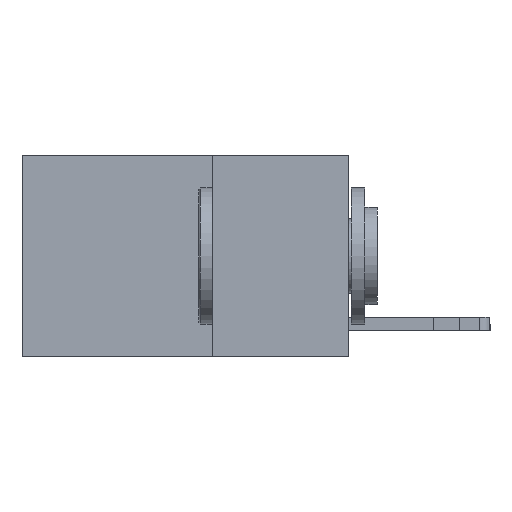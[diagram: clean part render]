
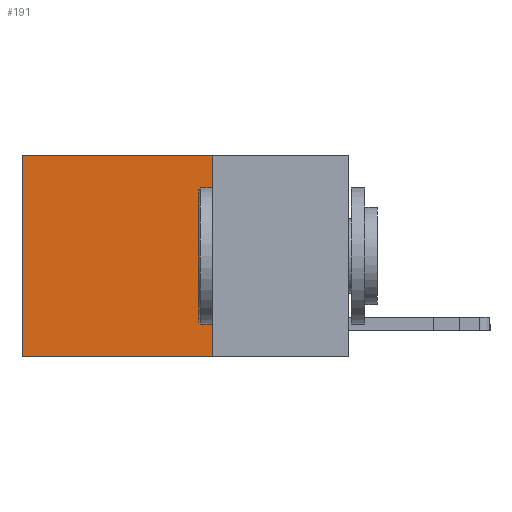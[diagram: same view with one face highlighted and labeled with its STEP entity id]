
A CAD part, left-side view. The second image highlights one B-rep face of the part: STEP entity #191.
In plain terms, the highlighted planar face has unit normal (-1, 0, 0).
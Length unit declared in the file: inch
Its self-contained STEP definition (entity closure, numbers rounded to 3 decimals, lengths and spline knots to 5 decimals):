
#33 = PLANE ( 'NONE',  #14821 ) ;
#191 = ADVANCED_FACE ( 'NONE', ( #10286 ), #33, .F. ) ;
#296 = CARTESIAN_POINT ( 'NONE',  ( 0.2625, 0.25, 0. ) ) ;
#1462 = DIRECTION ( 'NONE',  ( 0., 0., -1. ) ) ;
#2410 = CARTESIAN_POINT ( 'NONE',  ( 0.2625, 0.6, 0. ) ) ;
#2831 = DIRECTION ( 'NONE',  ( 0., 0., -1. ) ) ;
#4103 = CARTESIAN_POINT ( 'NONE',  ( 0.2625, 0.25, -0.37 ) ) ;
#4836 = ORIENTED_EDGE ( 'NONE', *, *, #6545, .F. ) ;
#4882 = DIRECTION ( 'NONE',  ( 1., 0., 0. ) ) ;
#6545 = EDGE_CURVE ( 'NONE', #16766, #10896, #7653, .T. ) ;
#7653 = LINE ( 'NONE', #4103, #22746 ) ;
#8190 = VECTOR ( 'NONE', #2831, 39.37008 ) ;
#8811 = CARTESIAN_POINT ( 'NONE',  ( 0.2625, 0.6, 0. ) ) ;
#8828 = ORIENTED_EDGE ( 'NONE', *, *, #20464, .T. ) ;
#9336 = CARTESIAN_POINT ( 'NONE',  ( 0.2625, 0.6, -0.37 ) ) ;
#9609 = CARTESIAN_POINT ( 'NONE',  ( 0.2625, 0.25, 0. ) ) ;
#9958 = LINE ( 'NONE', #9609, #13652 ) ;
#10286 = FACE_OUTER_BOUND ( 'NONE', #22119, .T. ) ;
#10896 = VERTEX_POINT ( 'NONE', #9336 ) ;
#12114 = VERTEX_POINT ( 'NONE', #296 ) ;
#12209 = LINE ( 'NONE', #8811, #22884 ) ;
#12689 = EDGE_CURVE ( 'NONE', #12114, #16766, #16728, .T. ) ;
#13377 = ORIENTED_EDGE ( 'NONE', *, *, #12689, .F. ) ;
#13652 = VECTOR ( 'NONE', #20210, 39.37008 ) ;
#14283 = CARTESIAN_POINT ( 'NONE',  ( 0.2625, 0.25, 0. ) ) ;
#14821 = AXIS2_PLACEMENT_3D ( 'NONE', #14283, #4882, #1462 ) ;
#16728 = LINE ( 'NONE', #20826, #8190 ) ;
#16766 = VERTEX_POINT ( 'NONE', #20077 ) ;
#17743 = DIRECTION ( 'NONE',  ( 0., 0., -1. ) ) ;
#19477 = ORIENTED_EDGE ( 'NONE', *, *, #21421, .T. ) ;
#20077 = CARTESIAN_POINT ( 'NONE',  ( 0.2625, 0.25, -0.37 ) ) ;
#20210 = DIRECTION ( 'NONE',  ( 0., 1., 0. ) ) ;
#20464 = EDGE_CURVE ( 'NONE', #12114, #22065, #9958, .T. ) ;
#20826 = CARTESIAN_POINT ( 'NONE',  ( 0.2625, 0.25, 0. ) ) ;
#21421 = EDGE_CURVE ( 'NONE', #22065, #10896, #12209, .T. ) ;
#22065 = VERTEX_POINT ( 'NONE', #2410 ) ;
#22119 = EDGE_LOOP ( 'NONE', ( #19477, #4836, #13377, #8828 ) ) ;
#22693 = DIRECTION ( 'NONE',  ( 0., 1., 0. ) ) ;
#22746 = VECTOR ( 'NONE', #22693, 39.37008 ) ;
#22884 = VECTOR ( 'NONE', #17743, 39.37008 ) ;
